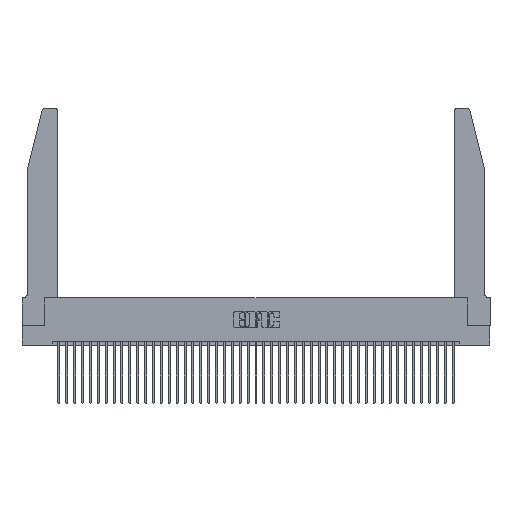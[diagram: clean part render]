
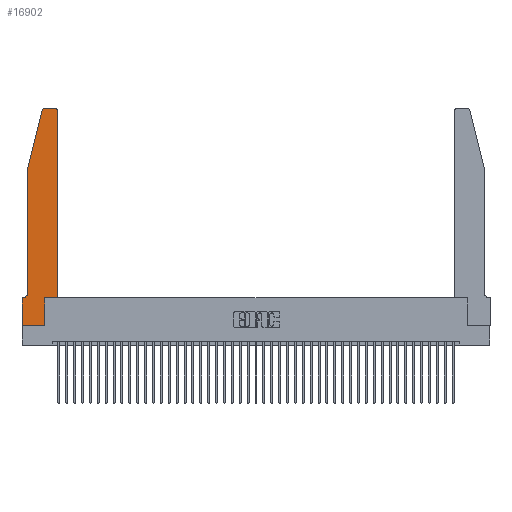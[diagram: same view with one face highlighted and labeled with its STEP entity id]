
A CAD part, top view. The second image highlights one B-rep face of the part: STEP entity #16902.
In plain terms, the highlighted planar face has unit normal (0, 0, 1).
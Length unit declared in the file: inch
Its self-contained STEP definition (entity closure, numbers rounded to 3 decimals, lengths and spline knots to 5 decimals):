
#194 = VERTEX_POINT ( 'NONE', #930 ) ;
#930 = CARTESIAN_POINT ( 'NONE',  ( 0.25487, 2.72718, 0.37 ) ) ;
#1045 = LINE ( 'NONE', #42620, #35812 ) ;
#1115 = DIRECTION ( 'NONE',  ( 1., 0., 0. ) ) ;
#1661 = VECTOR ( 'NONE', #18928, 39.37008 ) ;
#2948 = CARTESIAN_POINT ( 'NONE',  ( 0.2605, 2.75, 0.37 ) ) ;
#3332 = EDGE_CURVE ( 'NONE', #5017, #20626, #26253, .T. ) ;
#3883 = FACE_OUTER_BOUND ( 'NONE', #23017, .T. ) ;
#4411 = DIRECTION ( 'NONE',  ( -1., 0., 0. ) ) ;
#4512 = VERTEX_POINT ( 'NONE', #31366 ) ;
#4785 = ORIENTED_EDGE ( 'NONE', *, *, #18594, .T. ) ;
#5017 = VERTEX_POINT ( 'NONE', #15549 ) ;
#5332 = CARTESIAN_POINT ( 'NONE',  ( 0.0755, 2., 0.37 ) ) ;
#6083 = EDGE_CURVE ( 'NONE', #25641, #5017, #21079, .T. ) ;
#6724 = CARTESIAN_POINT ( 'NONE',  ( 0.284, 2.72, 0.37 ) ) ;
#7613 = VECTOR ( 'NONE', #20043, 39.37008 ) ;
#7880 = CARTESIAN_POINT ( 'NONE',  ( 0.2865, 0.35, 0.37 ) ) ;
#8054 = ORIENTED_EDGE ( 'NONE', *, *, #13398, .T. ) ;
#8322 = ORIENTED_EDGE ( 'NONE', *, *, #31973, .T. ) ;
#9134 = DIRECTION ( 'NONE',  ( 0., -1., 0. ) ) ;
#10137 = DIRECTION ( 'NONE',  ( 0., 0., 1. ) ) ;
#10161 = ORIENTED_EDGE ( 'NONE', *, *, #35188, .T. ) ;
#10405 = ORIENTED_EDGE ( 'NONE', *, *, #6083, .T. ) ;
#10513 = ORIENTED_EDGE ( 'NONE', *, *, #25822, .T. ) ;
#10655 = PLANE ( 'NONE',  #38507 ) ;
#10778 = CARTESIAN_POINT ( 'NONE',  ( 0.4505, 2.72, 0.37 ) ) ;
#11123 = CARTESIAN_POINT ( 'NONE',  ( 0.4205, 2.72, 0.37 ) ) ;
#11765 = CARTESIAN_POINT ( 'NONE',  ( 0.284, 2.75, 0.37 ) ) ;
#12393 = CARTESIAN_POINT ( 'NONE',  ( 0.2865, 0., 0.37 ) ) ;
#12515 = EDGE_CURVE ( 'NONE', #32193, #25641, #37481, .T. ) ;
#12842 = CARTESIAN_POINT ( 'NONE',  ( 0.0055, 0.35, 0.37 ) ) ;
#13125 = DIRECTION ( 'NONE',  ( -1., 0., 0. ) ) ;
#13396 = EDGE_CURVE ( 'NONE', #38966, #32193, #20051, .T. ) ;
#13398 = EDGE_CURVE ( 'NONE', #30961, #28040, #28463, .T. ) ;
#14175 = AXIS2_PLACEMENT_3D ( 'NONE', #31358, #20608, #4411 ) ;
#15549 = CARTESIAN_POINT ( 'NONE',  ( 0.4205, 2.75, 0.37 ) ) ;
#16902 = ADVANCED_FACE ( 'NONE', ( #3883 ), #10655, .T. ) ;
#17439 = DIRECTION ( 'NONE',  ( 0., 0., 1. ) ) ;
#17943 = VERTEX_POINT ( 'NONE', #12842 ) ;
#18548 = LINE ( 'NONE', #5332, #40617 ) ;
#18594 = EDGE_CURVE ( 'NONE', #194, #39969, #41453, .T. ) ;
#18881 = ORIENTED_EDGE ( 'NONE', *, *, #12515, .T. ) ;
#18928 = DIRECTION ( 'NONE',  ( 0., 1., 0. ) ) ;
#19508 = CARTESIAN_POINT ( 'NONE',  ( 0.4505, 0.35, 0.37 ) ) ;
#20043 = DIRECTION ( 'NONE',  ( -1., 0., 0. ) ) ;
#20051 = LINE ( 'NONE', #19508, #36949 ) ;
#20608 = DIRECTION ( 'NONE',  ( 0., 0., -1. ) ) ;
#20626 = VERTEX_POINT ( 'NONE', #11765 ) ;
#21079 = CIRCLE ( 'NONE', #41907, 0.03 ) ;
#21161 = DIRECTION ( 'NONE',  ( 0., 1., 0. ) ) ;
#21224 = ORIENTED_EDGE ( 'NONE', *, *, #24097, .T. ) ;
#22681 = VECTOR ( 'NONE', #23024, 39.37008 ) ;
#23017 = EDGE_LOOP ( 'NONE', ( #40803, #10161, #4785, #21224, #10513, #8322, #29172, #8054, #35197, #33171, #18881, #10405 ) ) ;
#23024 = DIRECTION ( 'NONE',  ( 1., 0., 0. ) ) ;
#23869 = AXIS2_PLACEMENT_3D ( 'NONE', #6724, #10137, #37260 ) ;
#23903 = CARTESIAN_POINT ( 'NONE',  ( 0.2865, 0.35, 0.37 ) ) ;
#24097 = EDGE_CURVE ( 'NONE', #39969, #4512, #18548, .T. ) ;
#24586 = CARTESIAN_POINT ( 'NONE',  ( 0.4505, 0.35, 0.37 ) ) ;
#25123 = VERTEX_POINT ( 'NONE', #40946 ) ;
#25641 = VERTEX_POINT ( 'NONE', #10778 ) ;
#25822 = EDGE_CURVE ( 'NONE', #4512, #17943, #38408, .T. ) ;
#25956 = DIRECTION ( 'NONE',  ( 0., -1., 0. ) ) ;
#26253 = LINE ( 'NONE', #2948, #36810 ) ;
#28040 = VERTEX_POINT ( 'NONE', #12393 ) ;
#28463 = LINE ( 'NONE', #36299, #22681 ) ;
#28980 = DIRECTION ( 'NONE',  ( -0.239, -0.971, 0. ) ) ;
#29172 = ORIENTED_EDGE ( 'NONE', *, *, #36336, .T. ) ;
#29940 = DIRECTION ( 'NONE',  ( 1., 0., 0. ) ) ;
#30961 = VERTEX_POINT ( 'NONE', #40224 ) ;
#31358 = CARTESIAN_POINT ( 'NONE',  ( 0.0055, 0.42, 0.37 ) ) ;
#31366 = CARTESIAN_POINT ( 'NONE',  ( 0.0755, 0.42, 0.37 ) ) ;
#31815 = CARTESIAN_POINT ( 'NONE',  ( 0.0755, 2., 0.37 ) ) ;
#31973 = EDGE_CURVE ( 'NONE', #17943, #25123, #38757, .T. ) ;
#31995 = LINE ( 'NONE', #7880, #43067 ) ;
#32193 = VERTEX_POINT ( 'NONE', #24586 ) ;
#32502 = VECTOR ( 'NONE', #28980, 39.37008 ) ;
#32667 = CARTESIAN_POINT ( 'NONE',  ( 0.0755, 2., 0.37 ) ) ;
#32743 = CARTESIAN_POINT ( 'NONE',  ( 0.4505, 0.35, 0.37 ) ) ;
#33171 = ORIENTED_EDGE ( 'NONE', *, *, #13396, .T. ) ;
#34215 = CARTESIAN_POINT ( 'NONE',  ( 0., 0.35, 0.37 ) ) ;
#35188 = EDGE_CURVE ( 'NONE', #20626, #194, #41166, .T. ) ;
#35197 = ORIENTED_EDGE ( 'NONE', *, *, #38322, .T. ) ;
#35812 = VECTOR ( 'NONE', #25956, 39.37008 ) ;
#36299 = CARTESIAN_POINT ( 'NONE',  ( 0., 0., 0.37 ) ) ;
#36336 = EDGE_CURVE ( 'NONE', #25123, #30961, #1045, .T. ) ;
#36709 = CARTESIAN_POINT ( 'NONE',  ( 0.0755, 0.35, 0.37 ) ) ;
#36810 = VECTOR ( 'NONE', #13125, 39.37008 ) ;
#36949 = VECTOR ( 'NONE', #29940, 39.37008 ) ;
#37260 = DIRECTION ( 'NONE',  ( 1., 0., 0. ) ) ;
#37481 = LINE ( 'NONE', #32743, #1661 ) ;
#38322 = EDGE_CURVE ( 'NONE', #28040, #38966, #31995, .T. ) ;
#38408 = CIRCLE ( 'NONE', #14175, 0.07 ) ;
#38507 = AXIS2_PLACEMENT_3D ( 'NONE', #34215, #17439, #38770 ) ;
#38757 = LINE ( 'NONE', #36709, #7613 ) ;
#38770 = DIRECTION ( 'NONE',  ( 1., 0., 0. ) ) ;
#38966 = VERTEX_POINT ( 'NONE', #23903 ) ;
#39969 = VERTEX_POINT ( 'NONE', #32667 ) ;
#40224 = CARTESIAN_POINT ( 'NONE',  ( 0., 0., 0.37 ) ) ;
#40617 = VECTOR ( 'NONE', #9134, 39.37008 ) ;
#40803 = ORIENTED_EDGE ( 'NONE', *, *, #3332, .T. ) ;
#40946 = CARTESIAN_POINT ( 'NONE',  ( 0., 0.35, 0.37 ) ) ;
#41166 = CIRCLE ( 'NONE', #23869, 0.03 ) ;
#41443 = DIRECTION ( 'NONE',  ( 0., 0., 1. ) ) ;
#41453 = LINE ( 'NONE', #31815, #32502 ) ;
#41907 = AXIS2_PLACEMENT_3D ( 'NONE', #11123, #41443, #1115 ) ;
#42620 = CARTESIAN_POINT ( 'NONE',  ( 0., 0., 0.37 ) ) ;
#43067 = VECTOR ( 'NONE', #21161, 39.37008 ) ;
